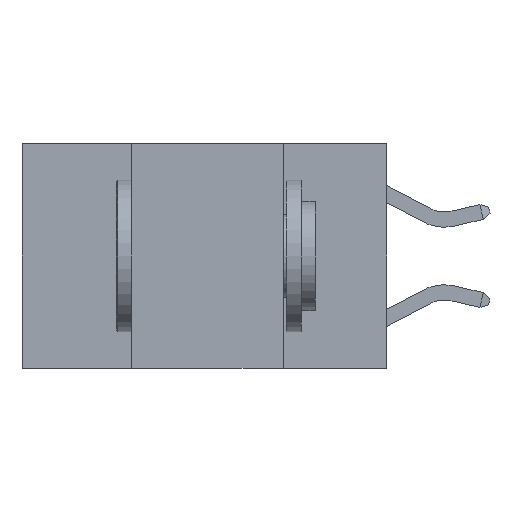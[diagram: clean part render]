
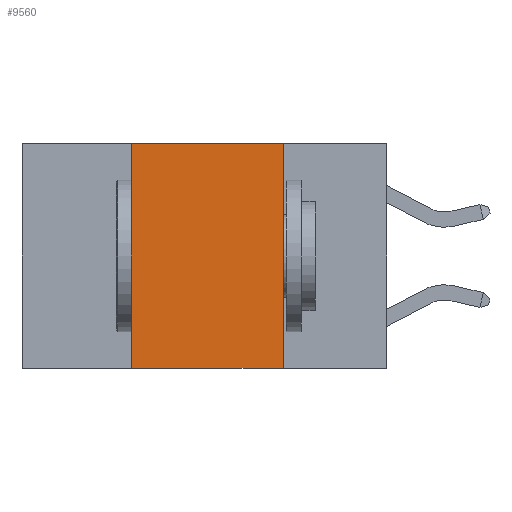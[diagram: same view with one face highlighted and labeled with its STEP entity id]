
A CAD part, left-side view. The second image highlights one B-rep face of the part: STEP entity #9560.
In plain terms, the highlighted planar face has unit normal (-1, 0, 0).
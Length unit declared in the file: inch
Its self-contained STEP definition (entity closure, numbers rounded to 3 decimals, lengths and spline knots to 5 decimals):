
#149 = CARTESIAN_POINT ( 'NONE',  ( 0., 0.17, 0. ) ) ;
#225 = CARTESIAN_POINT ( 'NONE',  ( 0., 0.42, 0. ) ) ;
#311 = DIRECTION ( 'NONE',  ( 0., -1., 0. ) ) ;
#412 = CARTESIAN_POINT ( 'NONE',  ( 0., 0.6, 0. ) ) ;
#542 = ORIENTED_EDGE ( 'NONE', *, *, #4082, .F. ) ;
#747 = EDGE_CURVE ( 'NONE', #10001, #2412, #5292, .T. ) ;
#802 = ORIENTED_EDGE ( 'NONE', *, *, #3826, .T. ) ;
#1690 = VECTOR ( 'NONE', #311, 39.37008 ) ;
#1982 = CARTESIAN_POINT ( 'NONE',  ( 0., 0.6, -0.37 ) ) ;
#1991 = DIRECTION ( 'NONE',  ( 0., -1., 0. ) ) ;
#2229 = AXIS2_PLACEMENT_3D ( 'NONE', #5291, #4493, #9944 ) ;
#2236 = VECTOR ( 'NONE', #3443, 39.37008 ) ;
#2412 = VERTEX_POINT ( 'NONE', #4259 ) ;
#2702 = ORIENTED_EDGE ( 'NONE', *, *, #9906, .F. ) ;
#3443 = DIRECTION ( 'NONE',  ( 0., 0., 1. ) ) ;
#3453 = VERTEX_POINT ( 'NONE', #5160 ) ;
#3628 = CARTESIAN_POINT ( 'NONE',  ( 0., 0.17, 0. ) ) ;
#3826 = EDGE_CURVE ( 'NONE', #3453, #2412, #10301, .T. ) ;
#4082 = EDGE_CURVE ( 'NONE', #8479, #10001, #8148, .T. ) ;
#4259 = CARTESIAN_POINT ( 'NONE',  ( 0., 0.17, -0.37 ) ) ;
#4317 = VECTOR ( 'NONE', #1991, 39.37008 ) ;
#4493 = DIRECTION ( 'NONE',  ( 1., 0., 0. ) ) ;
#4687 = ORIENTED_EDGE ( 'NONE', *, *, #747, .F. ) ;
#5160 = CARTESIAN_POINT ( 'NONE',  ( 0., 0.42, -0.37 ) ) ;
#5291 = CARTESIAN_POINT ( 'NONE',  ( 0., 0.6, 0. ) ) ;
#5292 = LINE ( 'NONE', #149, #9632 ) ;
#6671 = LINE ( 'NONE', #225, #2236 ) ;
#7243 = FACE_OUTER_BOUND ( 'NONE', #8706, .T. ) ;
#7667 = PLANE ( 'NONE',  #2229 ) ;
#8148 = LINE ( 'NONE', #412, #1690 ) ;
#8442 = CARTESIAN_POINT ( 'NONE',  ( 0., 0.42, 0. ) ) ;
#8479 = VERTEX_POINT ( 'NONE', #8442 ) ;
#8706 = EDGE_LOOP ( 'NONE', ( #4687, #542, #2702, #802 ) ) ;
#9560 = ADVANCED_FACE ( 'NONE', ( #7243 ), #7667, .F. ) ;
#9632 = VECTOR ( 'NONE', #10280, 39.37008 ) ;
#9906 = EDGE_CURVE ( 'NONE', #3453, #8479, #6671, .T. ) ;
#9944 = DIRECTION ( 'NONE',  ( 0., 0., -1. ) ) ;
#10001 = VERTEX_POINT ( 'NONE', #3628 ) ;
#10280 = DIRECTION ( 'NONE',  ( 0., 0., -1. ) ) ;
#10301 = LINE ( 'NONE', #1982, #4317 ) ;
